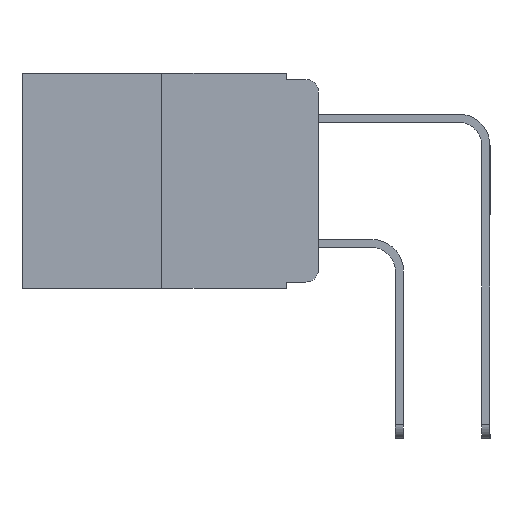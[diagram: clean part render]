
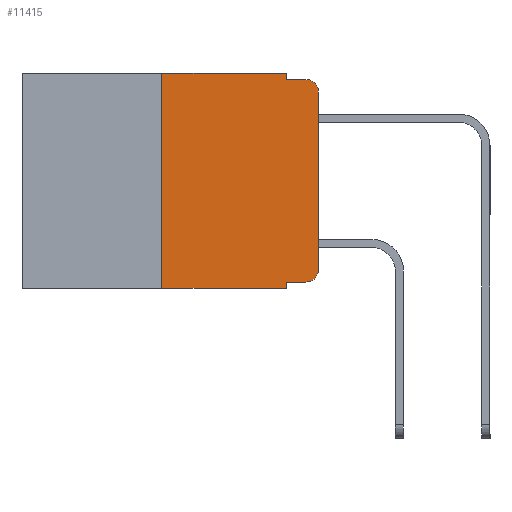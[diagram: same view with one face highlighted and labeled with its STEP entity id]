
A CAD part, left-side view. The second image highlights one B-rep face of the part: STEP entity #11415.
In plain terms, the highlighted planar face has unit normal (-1, 0, 0).
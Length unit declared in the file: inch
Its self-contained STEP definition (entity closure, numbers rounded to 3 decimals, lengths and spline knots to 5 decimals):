
#204 = ORIENTED_EDGE ( 'NONE', *, *, #9704, .F. ) ;
#446 = VECTOR ( 'NONE', #18999, 39.37008 ) ;
#462 = VERTEX_POINT ( 'NONE', #13004 ) ;
#473 = ORIENTED_EDGE ( 'NONE', *, *, #10877, .T. ) ;
#500 = ORIENTED_EDGE ( 'NONE', *, *, #7316, .F. ) ;
#1275 = VECTOR ( 'NONE', #9312, 39.37008 ) ;
#2113 = ORIENTED_EDGE ( 'NONE', *, *, #2398, .T. ) ;
#2398 = EDGE_CURVE ( 'NONE', #10212, #15138, #8026, .T. ) ;
#2688 = CARTESIAN_POINT ( 'NONE',  ( 0., 0.473, 0. ) ) ;
#4037 = DIRECTION ( 'NONE',  ( 0., -1., 0. ) ) ;
#4081 = VECTOR ( 'NONE', #7083, 39.37008 ) ;
#4169 = PLANE ( 'NONE',  #5740 ) ;
#4578 = CARTESIAN_POINT ( 'NONE',  ( 0., 0.02, -0.03 ) ) ;
#4826 = EDGE_CURVE ( 'NONE', #19273, #10212, #15217, .T. ) ;
#5664 = CARTESIAN_POINT ( 'NONE',  ( 0., 0.051, 0. ) ) ;
#5740 = AXIS2_PLACEMENT_3D ( 'NONE', #16428, #6010, #18188 ) ;
#5783 = VERTEX_POINT ( 'NONE', #12025 ) ;
#5890 = VERTEX_POINT ( 'NONE', #15654 ) ;
#6010 = DIRECTION ( 'NONE',  ( 1., 0., 0. ) ) ;
#6067 = EDGE_CURVE ( 'NONE', #19273, #15811, #14406, .T. ) ;
#6186 = DIRECTION ( 'NONE',  ( 0., 0., -1. ) ) ;
#6422 = DIRECTION ( 'NONE',  ( 0., 0., -1. ) ) ;
#6547 = ORIENTED_EDGE ( 'NONE', *, *, #21883, .T. ) ;
#6890 = CARTESIAN_POINT ( 'NONE',  ( 0., 0.473, -0.343 ) ) ;
#7083 = DIRECTION ( 'NONE',  ( 0., -1., 0. ) ) ;
#7232 = CARTESIAN_POINT ( 'NONE',  ( 0., 0.02, -0.333 ) ) ;
#7316 = EDGE_CURVE ( 'NONE', #20582, #13205, #7827, .T. ) ;
#7398 = ORIENTED_EDGE ( 'NONE', *, *, #11997, .T. ) ;
#7443 = EDGE_LOOP ( 'NONE', ( #7398, #473, #204, #11540, #16597, #500, #6547, #8837, #19045, #2113 ) ) ;
#7588 = AXIS2_PLACEMENT_3D ( 'NONE', #8379, #8256, #8325 ) ;
#7827 = LINE ( 'NONE', #11957, #13009 ) ;
#7911 = EDGE_CURVE ( 'NONE', #13205, #20847, #12543, .T. ) ;
#8026 = CIRCLE ( 'NONE', #7588, 0.02 ) ;
#8256 = DIRECTION ( 'NONE',  ( -1., 0., 0. ) ) ;
#8325 = DIRECTION ( 'NONE',  ( 0., 0., -1. ) ) ;
#8379 = CARTESIAN_POINT ( 'NONE',  ( 0., 0.02, -0.313 ) ) ;
#8489 = EDGE_CURVE ( 'NONE', #20847, #462, #10339, .T. ) ;
#8837 = ORIENTED_EDGE ( 'NONE', *, *, #6067, .F. ) ;
#8930 = LINE ( 'NONE', #15695, #4081 ) ;
#9312 = DIRECTION ( 'NONE',  ( 0., 0., -1. ) ) ;
#9704 = EDGE_CURVE ( 'NONE', #462, #5783, #8930, .T. ) ;
#10212 = VERTEX_POINT ( 'NONE', #7232 ) ;
#10213 = CARTESIAN_POINT ( 'NONE',  ( 0., 0.25, -0.343 ) ) ;
#10339 = LINE ( 'NONE', #18347, #14375 ) ;
#10512 = CARTESIAN_POINT ( 'NONE',  ( 0., 0.25, 0. ) ) ;
#10877 = EDGE_CURVE ( 'NONE', #5890, #5783, #12960, .T. ) ;
#11415 = ADVANCED_FACE ( 'NONE', ( #16365 ), #4169, .F. ) ;
#11540 = ORIENTED_EDGE ( 'NONE', *, *, #8489, .F. ) ;
#11786 = VECTOR ( 'NONE', #4037, 39.37008 ) ;
#11957 = CARTESIAN_POINT ( 'NONE',  ( 0., 0.25, 0. ) ) ;
#11997 = EDGE_CURVE ( 'NONE', #15138, #5890, #13994, .T. ) ;
#12025 = CARTESIAN_POINT ( 'NONE',  ( 0., 0.02, -0.01 ) ) ;
#12543 = LINE ( 'NONE', #2688, #21624 ) ;
#12960 = CIRCLE ( 'NONE', #14816, 0.02 ) ;
#13004 = CARTESIAN_POINT ( 'NONE',  ( 0., 0.051, -0.01 ) ) ;
#13009 = VECTOR ( 'NONE', #17092, 39.37008 ) ;
#13205 = VERTEX_POINT ( 'NONE', #10512 ) ;
#13779 = CARTESIAN_POINT ( 'NONE',  ( 0., 0., 0. ) ) ;
#13994 = LINE ( 'NONE', #13779, #22556 ) ;
#14375 = VECTOR ( 'NONE', #6186, 39.37008 ) ;
#14406 = LINE ( 'NONE', #5664, #1275 ) ;
#14816 = AXIS2_PLACEMENT_3D ( 'NONE', #4578, #16823, #6422 ) ;
#15138 = VERTEX_POINT ( 'NONE', #16439 ) ;
#15217 = LINE ( 'NONE', #18059, #11786 ) ;
#15654 = CARTESIAN_POINT ( 'NONE',  ( 0., 0., -0.03 ) ) ;
#15695 = CARTESIAN_POINT ( 'NONE',  ( 0., 0.051, -0.01 ) ) ;
#15811 = VERTEX_POINT ( 'NONE', #18379 ) ;
#16365 = FACE_OUTER_BOUND ( 'NONE', #7443, .T. ) ;
#16428 = CARTESIAN_POINT ( 'NONE',  ( 0., 0.473, 0. ) ) ;
#16439 = CARTESIAN_POINT ( 'NONE',  ( 0., 0., -0.313 ) ) ;
#16597 = ORIENTED_EDGE ( 'NONE', *, *, #7911, .F. ) ;
#16823 = DIRECTION ( 'NONE',  ( -1., 0., 0. ) ) ;
#17092 = DIRECTION ( 'NONE',  ( 0., 0., 1. ) ) ;
#18059 = CARTESIAN_POINT ( 'NONE',  ( 0., 0.051, -0.333 ) ) ;
#18083 = CARTESIAN_POINT ( 'NONE',  ( 0., 0.051, 0. ) ) ;
#18188 = DIRECTION ( 'NONE',  ( 0., 0., -1. ) ) ;
#18190 = LINE ( 'NONE', #6890, #446 ) ;
#18347 = CARTESIAN_POINT ( 'NONE',  ( 0., 0.051, 0. ) ) ;
#18379 = CARTESIAN_POINT ( 'NONE',  ( 0., 0.051, -0.343 ) ) ;
#18585 = DIRECTION ( 'NONE',  ( 0., -1., 0. ) ) ;
#18999 = DIRECTION ( 'NONE',  ( 0., -1., 0. ) ) ;
#19045 = ORIENTED_EDGE ( 'NONE', *, *, #4826, .T. ) ;
#19273 = VERTEX_POINT ( 'NONE', #20307 ) ;
#20307 = CARTESIAN_POINT ( 'NONE',  ( 0., 0.051, -0.333 ) ) ;
#20582 = VERTEX_POINT ( 'NONE', #10213 ) ;
#20847 = VERTEX_POINT ( 'NONE', #18083 ) ;
#21624 = VECTOR ( 'NONE', #18585, 39.37008 ) ;
#21883 = EDGE_CURVE ( 'NONE', #20582, #15811, #18190, .T. ) ;
#22361 = DIRECTION ( 'NONE',  ( 0., 0., 1. ) ) ;
#22556 = VECTOR ( 'NONE', #22361, 39.37008 ) ;
